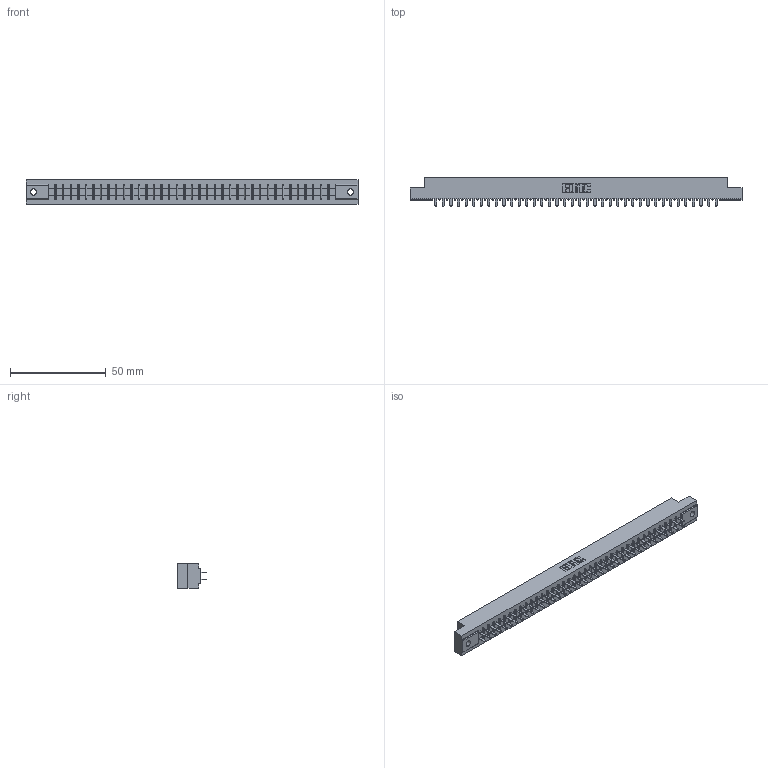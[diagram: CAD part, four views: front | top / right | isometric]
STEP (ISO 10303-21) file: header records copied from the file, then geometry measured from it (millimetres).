
FILE_DESCRIPTION (( 'STEP AP203' ), '1' );
FILE_NAME ('305-076-521-502.STEP', '2019-09-10T08:04:23', ( '' ), ( '' ), 'SwSTEP 2.0', 'SolidWorks 2016', '' );
FILE_SCHEMA (( 'CONFIG_CONTROL_DESIGN' ));
Length unit declared in the file: inch
Products named in the file (3): 305 Part_.128 Dia; 305-290-001_521; 305-076-521-502
Assembly tree (77 placements, depth 2):
  305-076-521-502
    305 Part_.128 Dia
    305-290-001_521  x76
Bounding box: 173.58 x 14.86 x 12.7 mm (x, y, z)
Volume: 17452.4 mm3; surface area: 22321.1 mm2
Topology: 77 solids, 77 shells, 3612 faces, 10310 edges, 6668 vertices
Faces by surface type: plane 2120, cylinder 1340, sphere 152
Entity records: 41513 total; most frequent: CARTESIAN_POINT 6868, ORIENTED_EDGE 6816, DIRECTION 6646, EDGE_CURVE 3408, LINE 2754, VECTOR 2754, VERTEX_POINT 2168, AXIS2_PLACEMENT_3D 1946
